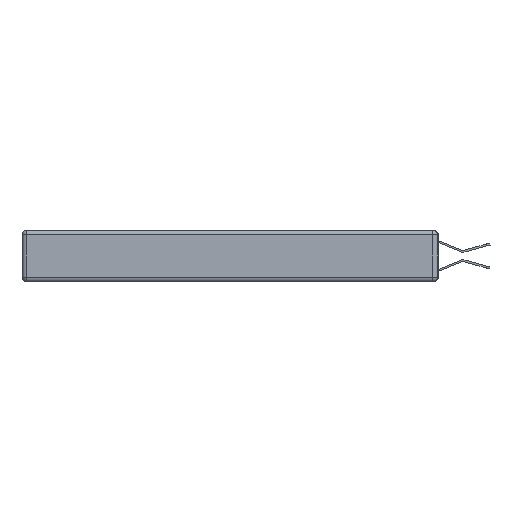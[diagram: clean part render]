
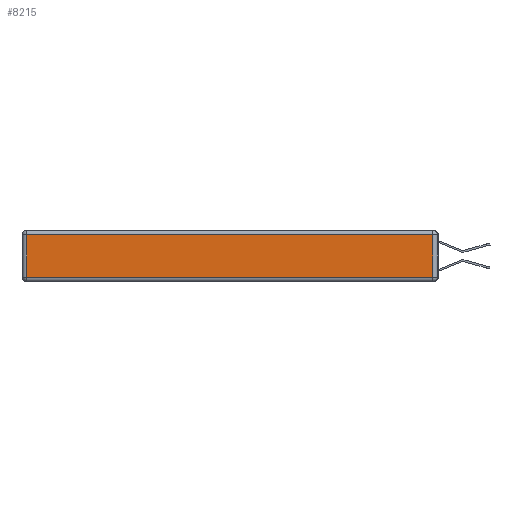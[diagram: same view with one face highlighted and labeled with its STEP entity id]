
A CAD part, left-side view. The second image highlights one B-rep face of the part: STEP entity #8215.
In plain terms, the highlighted planar face has unit normal (-1, 0, 0).
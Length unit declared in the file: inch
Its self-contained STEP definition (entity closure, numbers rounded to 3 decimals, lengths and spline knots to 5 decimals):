
#1036 = ORIENTED_EDGE ( 'NONE', *, *, #19876, .T. ) ;
#1289 = VECTOR ( 'NONE', #19157, 39.37008 ) ;
#2105 = ORIENTED_EDGE ( 'NONE', *, *, #6799, .T. ) ;
#2500 = VERTEX_POINT ( 'NONE', #10424 ) ;
#2767 = CARTESIAN_POINT ( 'NONE',  ( 0., 0.03, -0.343 ) ) ;
#2827 = CARTESIAN_POINT ( 'NONE',  ( 0., 0.03, -0.313 ) ) ;
#5110 = LINE ( 'NONE', #20472, #17136 ) ;
#5286 = CARTESIAN_POINT ( 'NONE',  ( 0., 2.75, -0.03 ) ) ;
#5382 = CARTESIAN_POINT ( 'NONE',  ( 0., 0., -0.343 ) ) ;
#5601 = DIRECTION ( 'NONE',  ( -1., 0., 0. ) ) ;
#6333 = DIRECTION ( 'NONE',  ( 0., 0., -1. ) ) ;
#6400 = LINE ( 'NONE', #2767, #1289 ) ;
#6799 = EDGE_CURVE ( 'NONE', #14646, #20093, #5110, .T. ) ;
#7303 = VECTOR ( 'NONE', #15319, 39.37008 ) ;
#8089 = EDGE_LOOP ( 'NONE', ( #2105, #14697, #1036, #14971 ) ) ;
#8215 = ADVANCED_FACE ( 'NONE', ( #14264 ), #15340, .T. ) ;
#10424 = CARTESIAN_POINT ( 'NONE',  ( 0., 2.72, -0.03 ) ) ;
#10890 = DIRECTION ( 'NONE',  ( 0., -1., 0. ) ) ;
#11719 = EDGE_CURVE ( 'NONE', #20093, #13470, #6400, .T. ) ;
#12014 = AXIS2_PLACEMENT_3D ( 'NONE', #5382, #5601, #16823 ) ;
#12383 = CARTESIAN_POINT ( 'NONE',  ( 0., 0.03, -0.03 ) ) ;
#13022 = CARTESIAN_POINT ( 'NONE',  ( 0., 2.72, -0.343 ) ) ;
#13470 = VERTEX_POINT ( 'NONE', #12383 ) ;
#14264 = FACE_OUTER_BOUND ( 'NONE', #8089, .T. ) ;
#14646 = VERTEX_POINT ( 'NONE', #15333 ) ;
#14697 = ORIENTED_EDGE ( 'NONE', *, *, #11719, .T. ) ;
#14971 = ORIENTED_EDGE ( 'NONE', *, *, #14991, .T. ) ;
#14991 = EDGE_CURVE ( 'NONE', #2500, #14646, #16204, .T. ) ;
#15319 = DIRECTION ( 'NONE',  ( 0., 1., 0. ) ) ;
#15333 = CARTESIAN_POINT ( 'NONE',  ( 0., 2.72, -0.313 ) ) ;
#15340 = PLANE ( 'NONE',  #12014 ) ;
#16204 = LINE ( 'NONE', #13022, #18261 ) ;
#16823 = DIRECTION ( 'NONE',  ( 0., 0., 1. ) ) ;
#17136 = VECTOR ( 'NONE', #10890, 39.37008 ) ;
#17270 = LINE ( 'NONE', #5286, #7303 ) ;
#18261 = VECTOR ( 'NONE', #6333, 39.37008 ) ;
#19157 = DIRECTION ( 'NONE',  ( 0., 0., 1. ) ) ;
#19876 = EDGE_CURVE ( 'NONE', #13470, #2500, #17270, .T. ) ;
#20093 = VERTEX_POINT ( 'NONE', #2827 ) ;
#20472 = CARTESIAN_POINT ( 'NONE',  ( 0., 0., -0.313 ) ) ;
